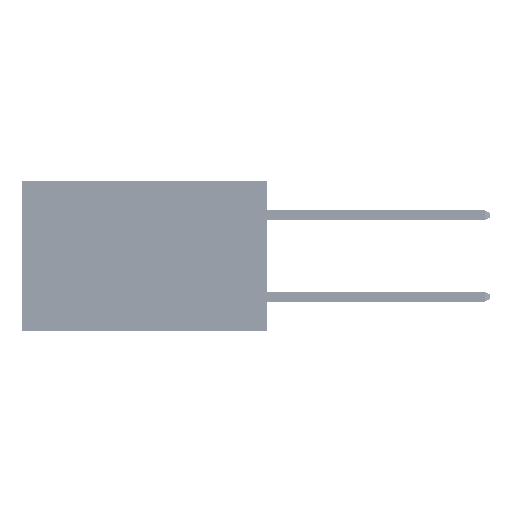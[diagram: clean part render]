
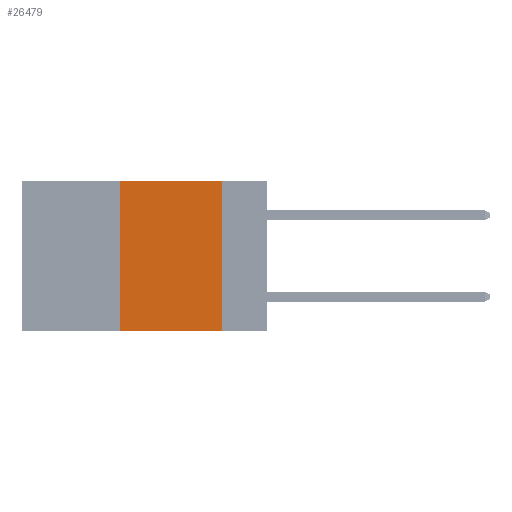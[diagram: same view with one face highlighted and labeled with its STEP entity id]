
A CAD part, left-side view. The second image highlights one B-rep face of the part: STEP entity #26479.
In plain terms, the highlighted planar face has unit normal (-1, 0, 0).
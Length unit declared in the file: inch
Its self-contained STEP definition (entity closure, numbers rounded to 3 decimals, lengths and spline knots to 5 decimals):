
#1552 = EDGE_CURVE ( 'NONE', #41066, #16377, #2357, .T. ) ;
#2357 = LINE ( 'NONE', #2602, #23343 ) ;
#2602 = CARTESIAN_POINT ( 'NONE',  ( 0., 0.36, 0. ) ) ;
#3035 = CARTESIAN_POINT ( 'NONE',  ( 0., 0.6, 0. ) ) ;
#6526 = LINE ( 'NONE', #3035, #38255 ) ;
#7392 = DIRECTION ( 'NONE',  ( 0., -1., 0. ) ) ;
#9121 = EDGE_CURVE ( 'NONE', #16377, #28306, #6526, .T. ) ;
#11218 = ORIENTED_EDGE ( 'NONE', *, *, #31935, .T. ) ;
#11379 = CARTESIAN_POINT ( 'NONE',  ( 0., 0.6, -0.37 ) ) ;
#12428 = DIRECTION ( 'NONE',  ( 1., 0., 0. ) ) ;
#15589 = LINE ( 'NONE', #11379, #25584 ) ;
#16377 = VERTEX_POINT ( 'NONE', #34554 ) ;
#16643 = ORIENTED_EDGE ( 'NONE', *, *, #9121, .F. ) ;
#17627 = ORIENTED_EDGE ( 'NONE', *, *, #26829, .F. ) ;
#19631 = VECTOR ( 'NONE', #29300, 39.37008 ) ;
#20372 = FACE_OUTER_BOUND ( 'NONE', #31604, .T. ) ;
#23343 = VECTOR ( 'NONE', #24497, 39.37008 ) ;
#24497 = DIRECTION ( 'NONE',  ( 0., 0., 1. ) ) ;
#25584 = VECTOR ( 'NONE', #7392, 39.37008 ) ;
#26479 = ADVANCED_FACE ( 'NONE', ( #20372 ), #27573, .F. ) ;
#26829 = EDGE_CURVE ( 'NONE', #28306, #39992, #41012, .T. ) ;
#27573 = PLANE ( 'NONE',  #43798 ) ;
#28306 = VERTEX_POINT ( 'NONE', #35475 ) ;
#29300 = DIRECTION ( 'NONE',  ( 0., 0., -1. ) ) ;
#31604 = EDGE_LOOP ( 'NONE', ( #17627, #16643, #32888, #11218 ) ) ;
#31935 = EDGE_CURVE ( 'NONE', #41066, #39992, #15589, .T. ) ;
#32888 = ORIENTED_EDGE ( 'NONE', *, *, #1552, .F. ) ;
#33214 = CARTESIAN_POINT ( 'NONE',  ( 0., 0.11, -0.37 ) ) ;
#33534 = CARTESIAN_POINT ( 'NONE',  ( 0., 0.11, 0. ) ) ;
#34554 = CARTESIAN_POINT ( 'NONE',  ( 0., 0.36, 0. ) ) ;
#35275 = DIRECTION ( 'NONE',  ( 0., 0., -1. ) ) ;
#35475 = CARTESIAN_POINT ( 'NONE',  ( 0., 0.11, 0. ) ) ;
#38255 = VECTOR ( 'NONE', #48573, 39.37008 ) ;
#39992 = VERTEX_POINT ( 'NONE', #33214 ) ;
#41012 = LINE ( 'NONE', #33534, #19631 ) ;
#41066 = VERTEX_POINT ( 'NONE', #45976 ) ;
#42067 = CARTESIAN_POINT ( 'NONE',  ( 0., 0.6, 0. ) ) ;
#43798 = AXIS2_PLACEMENT_3D ( 'NONE', #42067, #12428, #35275 ) ;
#45976 = CARTESIAN_POINT ( 'NONE',  ( 0., 0.36, -0.37 ) ) ;
#48573 = DIRECTION ( 'NONE',  ( 0., -1., 0. ) ) ;
